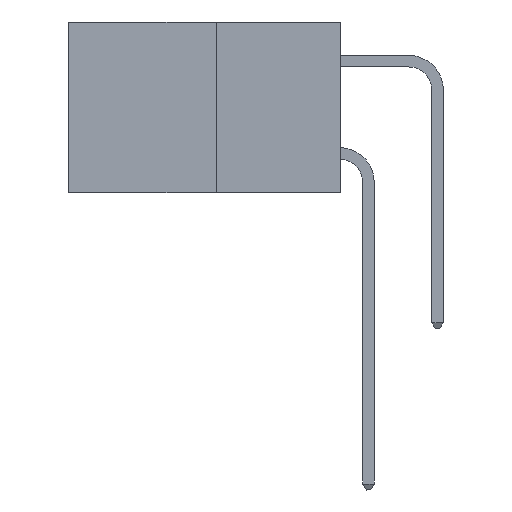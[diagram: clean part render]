
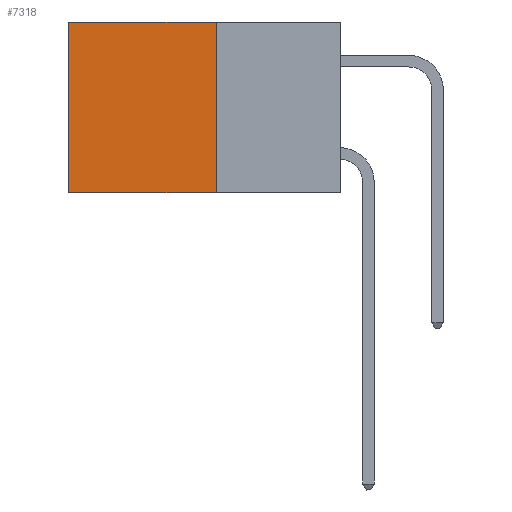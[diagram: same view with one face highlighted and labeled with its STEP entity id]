
A CAD part, left-side view. The second image highlights one B-rep face of the part: STEP entity #7318.
In plain terms, the highlighted planar face has unit normal (-1, 0, 0).
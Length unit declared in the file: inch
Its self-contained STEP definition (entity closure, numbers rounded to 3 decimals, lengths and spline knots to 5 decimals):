
#214 = VECTOR ( 'NONE', #2156, 39.37008 ) ;
#1994 = LINE ( 'NONE', #16442, #13581 ) ;
#2054 = ORIENTED_EDGE ( 'NONE', *, *, #13733, .F. ) ;
#2156 = DIRECTION ( 'NONE',  ( 0., 1., 0. ) ) ;
#2496 = ORIENTED_EDGE ( 'NONE', *, *, #11471, .F. ) ;
#2988 = DIRECTION ( 'NONE',  ( 0., 1., 0. ) ) ;
#3065 = CARTESIAN_POINT ( 'NONE',  ( 0.277, 0.59, -0.37 ) ) ;
#3398 = EDGE_CURVE ( 'NONE', #7603, #18975, #5639, .T. ) ;
#3451 = EDGE_LOOP ( 'NONE', ( #11683, #2496, #2054, #10770 ) ) ;
#4714 = LINE ( 'NONE', #9678, #214 ) ;
#4945 = CARTESIAN_POINT ( 'NONE',  ( 0.277, 0.27, 0. ) ) ;
#5639 = LINE ( 'NONE', #4945, #13191 ) ;
#6634 = PLANE ( 'NONE',  #13479 ) ;
#7318 = ADVANCED_FACE ( 'NONE', ( #8573 ), #6634, .F. ) ;
#7603 = VERTEX_POINT ( 'NONE', #13294 ) ;
#7818 = VERTEX_POINT ( 'NONE', #13800 ) ;
#8573 = FACE_OUTER_BOUND ( 'NONE', #3451, .T. ) ;
#9651 = DIRECTION ( 'NONE',  ( 0., 0., -1. ) ) ;
#9678 = CARTESIAN_POINT ( 'NONE',  ( 0.277, 0.27, -0.37 ) ) ;
#10770 = ORIENTED_EDGE ( 'NONE', *, *, #3398, .T. ) ;
#11186 = VERTEX_POINT ( 'NONE', #3065 ) ;
#11471 = EDGE_CURVE ( 'NONE', #7818, #11186, #4714, .T. ) ;
#11683 = ORIENTED_EDGE ( 'NONE', *, *, #15978, .T. ) ;
#11739 = LINE ( 'NONE', #15867, #19167 ) ;
#12925 = DIRECTION ( 'NONE',  ( 0., 0., -1. ) ) ;
#13191 = VECTOR ( 'NONE', #2988, 39.37008 ) ;
#13294 = CARTESIAN_POINT ( 'NONE',  ( 0.277, 0.27, 0. ) ) ;
#13479 = AXIS2_PLACEMENT_3D ( 'NONE', #17148, #18619, #9651 ) ;
#13509 = DIRECTION ( 'NONE',  ( 0., 0., -1. ) ) ;
#13581 = VECTOR ( 'NONE', #13509, 39.37008 ) ;
#13733 = EDGE_CURVE ( 'NONE', #7603, #7818, #11739, .T. ) ;
#13800 = CARTESIAN_POINT ( 'NONE',  ( 0.277, 0.27, -0.37 ) ) ;
#15688 = CARTESIAN_POINT ( 'NONE',  ( 0.277, 0.59, 0. ) ) ;
#15867 = CARTESIAN_POINT ( 'NONE',  ( 0.277, 0.27, -0.37 ) ) ;
#15978 = EDGE_CURVE ( 'NONE', #18975, #11186, #1994, .T. ) ;
#16442 = CARTESIAN_POINT ( 'NONE',  ( 0.277, 0.59, -0.37 ) ) ;
#17148 = CARTESIAN_POINT ( 'NONE',  ( 0.277, 0.27, -0.37 ) ) ;
#18619 = DIRECTION ( 'NONE',  ( 1., 0., 0. ) ) ;
#18975 = VERTEX_POINT ( 'NONE', #15688 ) ;
#19167 = VECTOR ( 'NONE', #12925, 39.37008 ) ;
